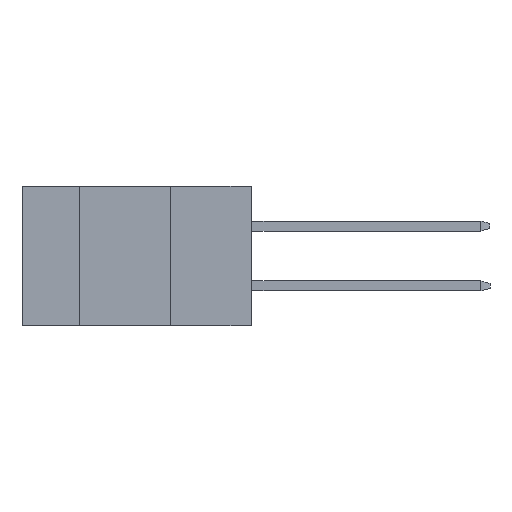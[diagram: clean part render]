
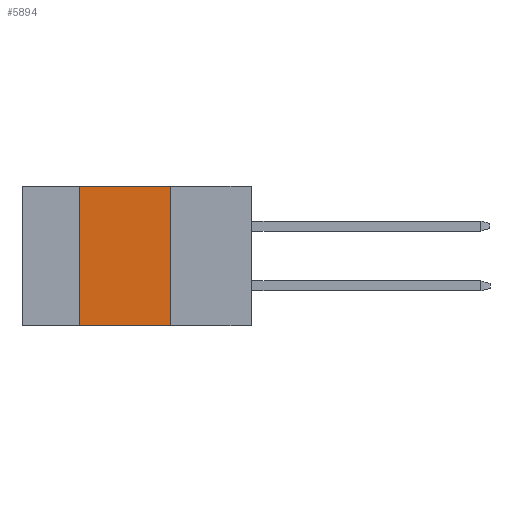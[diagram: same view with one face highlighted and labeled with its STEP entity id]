
A CAD part, left-side view. The second image highlights one B-rep face of the part: STEP entity #5894.
In plain terms, the highlighted planar face has unit normal (-1, 0, 0).
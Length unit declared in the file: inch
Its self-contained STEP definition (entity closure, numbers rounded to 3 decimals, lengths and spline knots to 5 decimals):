
#420 = ORIENTED_EDGE ( 'NONE', *, *, #5152, .F. ) ;
#583 = EDGE_LOOP ( 'NONE', ( #18952, #420, #17148, #8159 ) ) ;
#1673 = LINE ( 'NONE', #17397, #19582 ) ;
#1780 = DIRECTION ( 'NONE',  ( 0., -1., 0. ) ) ;
#4105 = DIRECTION ( 'NONE',  ( 0., 0., -1. ) ) ;
#4300 = CARTESIAN_POINT ( 'NONE',  ( 0., 0.254, 0. ) ) ;
#4562 = AXIS2_PLACEMENT_3D ( 'NONE', #19707, #11878, #4105 ) ;
#5152 = EDGE_CURVE ( 'NONE', #11563, #11614, #1673, .T. ) ;
#5626 = FACE_OUTER_BOUND ( 'NONE', #583, .T. ) ;
#5689 = CARTESIAN_POINT ( 'NONE',  ( 0., 0.254, -0.437 ) ) ;
#5894 = ADVANCED_FACE ( 'NONE', ( #5626 ), #19605, .F. ) ;
#8159 = ORIENTED_EDGE ( 'NONE', *, *, #16375, .T. ) ;
#9118 = VERTEX_POINT ( 'NONE', #14634 ) ;
#9998 = CARTESIAN_POINT ( 'NONE',  ( 0., 0.72, -0.437 ) ) ;
#10109 = EDGE_CURVE ( 'NONE', #11614, #9118, #10393, .T. ) ;
#10393 = LINE ( 'NONE', #5689, #18799 ) ;
#10474 = CARTESIAN_POINT ( 'NONE',  ( 0., 0.54, -0.437 ) ) ;
#10597 = VECTOR ( 'NONE', #12324, 39.37008 ) ;
#10619 = EDGE_CURVE ( 'NONE', #18903, #11563, #13846, .T. ) ;
#11563 = VERTEX_POINT ( 'NONE', #16642 ) ;
#11614 = VERTEX_POINT ( 'NONE', #4300 ) ;
#11878 = DIRECTION ( 'NONE',  ( 1., 0., 0. ) ) ;
#12324 = DIRECTION ( 'NONE',  ( 0., 0., 1. ) ) ;
#13159 = CARTESIAN_POINT ( 'NONE',  ( 0., 0.54, -0.437 ) ) ;
#13846 = LINE ( 'NONE', #10474, #10597 ) ;
#14634 = CARTESIAN_POINT ( 'NONE',  ( 0., 0.254, -0.437 ) ) ;
#14914 = DIRECTION ( 'NONE',  ( 0., -1., 0. ) ) ;
#16375 = EDGE_CURVE ( 'NONE', #18903, #9118, #18908, .T. ) ;
#16642 = CARTESIAN_POINT ( 'NONE',  ( 0., 0.54, 0. ) ) ;
#17148 = ORIENTED_EDGE ( 'NONE', *, *, #10619, .F. ) ;
#17397 = CARTESIAN_POINT ( 'NONE',  ( 0., 0.72, 0. ) ) ;
#18333 = VECTOR ( 'NONE', #14914, 39.37008 ) ;
#18799 = VECTOR ( 'NONE', #19574, 39.37008 ) ;
#18903 = VERTEX_POINT ( 'NONE', #13159 ) ;
#18908 = LINE ( 'NONE', #9998, #18333 ) ;
#18952 = ORIENTED_EDGE ( 'NONE', *, *, #10109, .F. ) ;
#19574 = DIRECTION ( 'NONE',  ( 0., 0., -1. ) ) ;
#19582 = VECTOR ( 'NONE', #1780, 39.37008 ) ;
#19605 = PLANE ( 'NONE',  #4562 ) ;
#19707 = CARTESIAN_POINT ( 'NONE',  ( 0., 0.72, 0. ) ) ;
